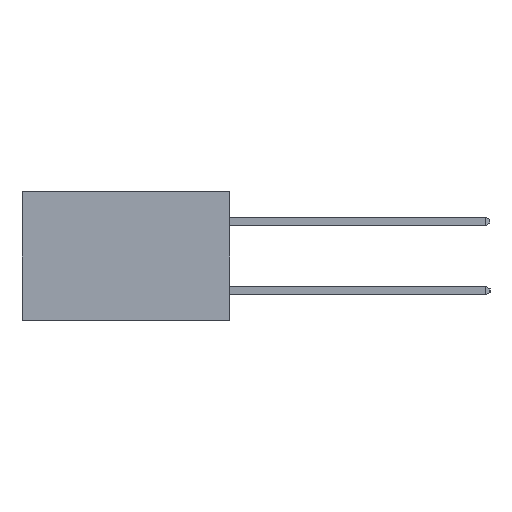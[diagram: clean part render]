
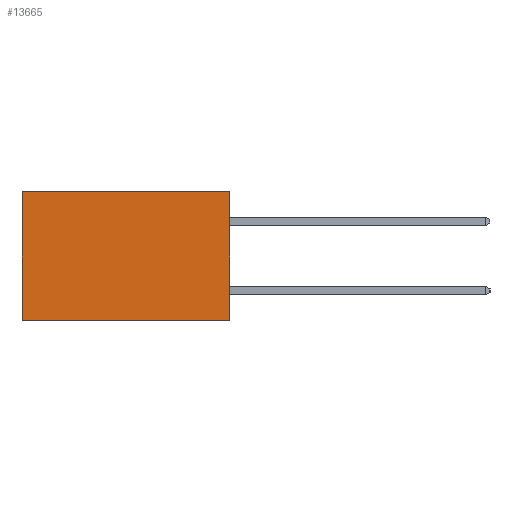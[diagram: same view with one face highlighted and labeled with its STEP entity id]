
A CAD part, left-side view. The second image highlights one B-rep face of the part: STEP entity #13665.
In plain terms, the highlighted planar face has unit normal (-1, 0, 0).
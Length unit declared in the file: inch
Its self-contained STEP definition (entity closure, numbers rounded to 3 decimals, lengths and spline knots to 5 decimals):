
#506 = FACE_OUTER_BOUND ( 'NONE', #937, .T. ) ;
#583 = CARTESIAN_POINT ( 'NONE',  ( 0.2615, 0.6, 0. ) ) ;
#777 = EDGE_CURVE ( 'NONE', #16373, #5355, #6050, .T. ) ;
#937 = EDGE_LOOP ( 'NONE', ( #12486, #12130, #14820, #17502 ) ) ;
#1089 = CARTESIAN_POINT ( 'NONE',  ( 0.2615, 0.6, -0.37 ) ) ;
#1993 = CARTESIAN_POINT ( 'NONE',  ( 0.2615, 0., -0.37 ) ) ;
#2665 = CARTESIAN_POINT ( 'NONE',  ( 0.2615, 0., 0. ) ) ;
#2779 = CARTESIAN_POINT ( 'NONE',  ( 0.2615, 0., -0.37 ) ) ;
#2926 = CARTESIAN_POINT ( 'NONE',  ( 0.2615, 0., -0.37 ) ) ;
#3083 = DIRECTION ( 'NONE',  ( 0., 1., 0. ) ) ;
#4107 = EDGE_CURVE ( 'NONE', #15408, #7344, #14324, .T. ) ;
#5355 = VERTEX_POINT ( 'NONE', #1089 ) ;
#6050 = LINE ( 'NONE', #2926, #16250 ) ;
#6065 = VECTOR ( 'NONE', #6429, 39.37008 ) ;
#6417 = VECTOR ( 'NONE', #16294, 39.37008 ) ;
#6429 = DIRECTION ( 'NONE',  ( 0., 0., -1. ) ) ;
#6482 = DIRECTION ( 'NONE',  ( 1., 0., 0. ) ) ;
#7000 = AXIS2_PLACEMENT_3D ( 'NONE', #14480, #6482, #15805 ) ;
#7344 = VERTEX_POINT ( 'NONE', #583 ) ;
#9184 = PLANE ( 'NONE',  #7000 ) ;
#10844 = VECTOR ( 'NONE', #11232, 39.37008 ) ;
#11232 = DIRECTION ( 'NONE',  ( 0., 1., 0. ) ) ;
#12130 = ORIENTED_EDGE ( 'NONE', *, *, #777, .F. ) ;
#12188 = EDGE_CURVE ( 'NONE', #7344, #5355, #16655, .T. ) ;
#12486 = ORIENTED_EDGE ( 'NONE', *, *, #12188, .T. ) ;
#13118 = CARTESIAN_POINT ( 'NONE',  ( 0.2615, 0.6, -0.37 ) ) ;
#13665 = ADVANCED_FACE ( 'NONE', ( #506 ), #9184, .F. ) ;
#13946 = EDGE_CURVE ( 'NONE', #15408, #16373, #13968, .T. ) ;
#13968 = LINE ( 'NONE', #2779, #6417 ) ;
#14068 = CARTESIAN_POINT ( 'NONE',  ( 0.2615, 0., 0. ) ) ;
#14324 = LINE ( 'NONE', #14068, #10844 ) ;
#14480 = CARTESIAN_POINT ( 'NONE',  ( 0.2615, 0., -0.37 ) ) ;
#14820 = ORIENTED_EDGE ( 'NONE', *, *, #13946, .F. ) ;
#15408 = VERTEX_POINT ( 'NONE', #2665 ) ;
#15805 = DIRECTION ( 'NONE',  ( 0., 0., -1. ) ) ;
#16250 = VECTOR ( 'NONE', #3083, 39.37008 ) ;
#16294 = DIRECTION ( 'NONE',  ( 0., 0., -1. ) ) ;
#16373 = VERTEX_POINT ( 'NONE', #1993 ) ;
#16655 = LINE ( 'NONE', #13118, #6065 ) ;
#17502 = ORIENTED_EDGE ( 'NONE', *, *, #4107, .T. ) ;
